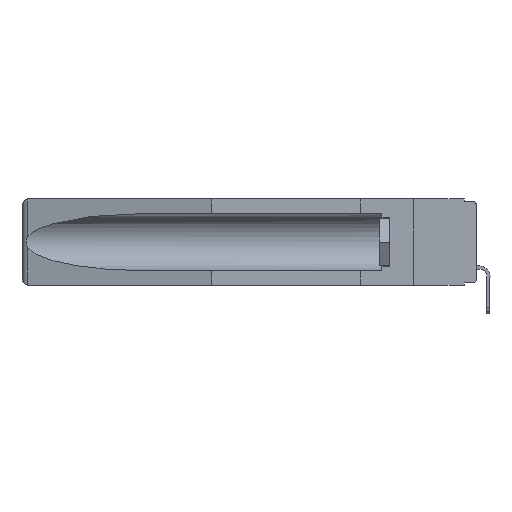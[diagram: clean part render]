
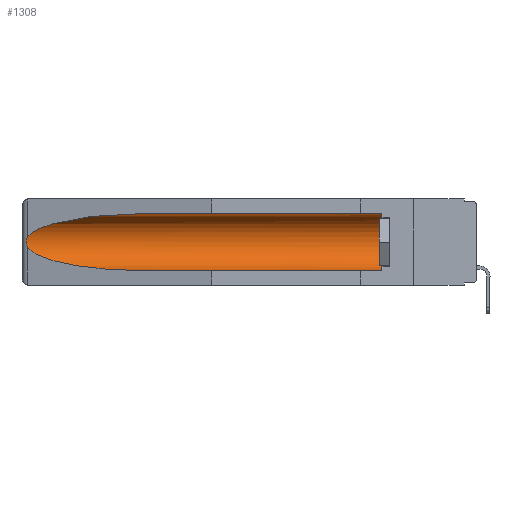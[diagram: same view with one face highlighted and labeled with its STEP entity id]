
A CAD part, left-side view. The second image highlights one B-rep face of the part: STEP entity #1308.
In plain terms, the highlighted cylindrical face has radius 2.857 mm (diameter 5.715 mm), a partial arc.
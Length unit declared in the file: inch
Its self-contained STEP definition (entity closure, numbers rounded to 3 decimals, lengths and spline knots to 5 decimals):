
#614 = ORIENTED_EDGE ( 'NONE', *, *, #19850, .T. ) ;
#837 = CARTESIAN_POINT ( 'NONE',  ( 0.26537, 1.52718, -0.19328 ) ) ;
#1308 = ADVANCED_FACE ( 'NONE', ( #6739 ), #22588, .F. ) ;
#1332 = EDGE_LOOP ( 'NONE', ( #6736, #7209, #614, #4670, #7236, #24581 ) ) ;
#2397 = VERTEX_POINT ( 'NONE', #21921 ) ;
#3023 = DIRECTION ( 'NONE',  ( 0., 0., 1. ) ) ;
#3344 = CARTESIAN_POINT ( 'NONE',  ( 0.155, 1.07973, -0.284 ) ) ;
#3628 = CARTESIAN_POINT ( 'NONE',  ( 0.21114, 1.30732, -0.284 ) ) ;
#4670 = ORIENTED_EDGE ( 'NONE', *, *, #9029, .F. ) ;
#4685 = AXIS2_PLACEMENT_3D ( 'NONE', #4795, #16959, #17043 ) ;
#4795 = CARTESIAN_POINT ( 'NONE',  ( 0.155, -0.30754, -0.1715 ) ) ;
#4807 = CARTESIAN_POINT ( 'NONE',  ( 0.26654, 1.53092, -0.15636 ) ) ;
#5540 = CARTESIAN_POINT ( 'NONE',  ( 0.155, 1.07973, -0.059 ) ) ;
#6115 = AXIS2_PLACEMENT_3D ( 'NONE', #7276, #15375, #3023 ) ;
#6623 = CARTESIAN_POINT ( 'NONE',  ( 0.26537, 1.52718, -0.14972 ) ) ;
#6736 = ORIENTED_EDGE ( 'NONE', *, *, #7638, .T. ) ;
#6739 = FACE_OUTER_BOUND ( 'NONE', #1332, .T. ) ;
#7209 = ORIENTED_EDGE ( 'NONE', *, *, #9747, .T. ) ;
#7236 = ORIENTED_EDGE ( 'NONE', *, *, #12128, .T. ) ;
#7238 = CARTESIAN_POINT ( 'NONE',  ( 0.155, 0.126, -0.059 ) ) ;
#7276 = CARTESIAN_POINT ( 'NONE',  ( 0.155, 0.126, -0.1715 ) ) ;
#7638 = EDGE_CURVE ( 'NONE', #10505, #26448, #10097, .T. ) ;
#7730 = VECTOR ( 'NONE', #8351, 39.37008 ) ;
#8350 = LINE ( 'NONE', #12063, #7730 ) ;
#8351 = DIRECTION ( 'NONE',  ( 0., 1., 0. ) ) ;
#8449 = CARTESIAN_POINT ( 'NONE',  ( 0.155, 1.07973, -0.284 ) ) ;
#9019 = VERTEX_POINT ( 'NONE', #7238 ) ;
#9029 = EDGE_CURVE ( 'NONE', #10270, #26548, #25011, .T. ) ;
#9129 = CARTESIAN_POINT ( 'NONE',  ( 0.26537, 1.52718, -0.14972 ) ) ;
#9357 = CARTESIAN_POINT ( 'NONE',  ( 0.21114, 1.30732, -0.059 ) ) ;
#9747 = EDGE_CURVE ( 'NONE', #26448, #2397, #12850, .T. ) ;
#9941 = CARTESIAN_POINT ( 'NONE',  ( 0.26537, 1.52718, -0.19328 ) ) ;
#10097 =( BOUNDED_CURVE ( )  B_SPLINE_CURVE ( 3, ( #17455, #9357, #14654, #6623 ),
 .UNSPECIFIED., .F., .T. ) 
 B_SPLINE_CURVE_WITH_KNOTS ( ( 4, 4 ),
 ( 4.71239, 6.08839 ),
 .UNSPECIFIED. ) 
 CURVE ( )  GEOMETRIC_REPRESENTATION_ITEM ( )  RATIONAL_B_SPLINE_CURVE ( ( 1., 0.848, 0.848, 1. ) ) 
 REPRESENTATION_ITEM ( '' )  );
#10270 = VERTEX_POINT ( 'NONE', #26228 ) ;
#10505 = VERTEX_POINT ( 'NONE', #5540 ) ;
#10785 = VECTOR ( 'NONE', #12995, 39.37008 ) ;
#10867 = CARTESIAN_POINT ( 'NONE',  ( 0.26655, 1.53094, -0.18657 ) ) ;
#12063 = CARTESIAN_POINT ( 'NONE',  ( 0.155, -0.30754, -0.059 ) ) ;
#12128 = EDGE_CURVE ( 'NONE', #10270, #9019, #15611, .T. ) ;
#12850 = B_SPLINE_CURVE_WITH_KNOTS ( 'NONE', 3,
 ( #9129, #23592, #4807, #25705, #13278, #13187, #21618, #10867, #25335, #837 ),
 .UNSPECIFIED., .F., .F.,
 ( 4, 2, 2, 2, 4 ),
 ( 0., 0.00029, 0.00058, 0.00087, 0.00117 ),
 .UNSPECIFIED. ) ;
#12995 = DIRECTION ( 'NONE',  ( 0., 1., 0. ) ) ;
#13187 = CARTESIAN_POINT ( 'NONE',  ( 0.2675, 1.53308, -0.17534 ) ) ;
#13278 = CARTESIAN_POINT ( 'NONE',  ( 0.2675, 1.53308, -0.16763 ) ) ;
#14654 = CARTESIAN_POINT ( 'NONE',  ( 0.25451, 1.48313, -0.09465 ) ) ;
#15375 = DIRECTION ( 'NONE',  ( 0., -1., 0. ) ) ;
#15611 = CIRCLE ( 'NONE', #6115, 0.1125 ) ;
#15881 = EDGE_CURVE ( 'NONE', #9019, #10505, #8350, .T. ) ;
#15953 = CARTESIAN_POINT ( 'NONE',  ( 0.25451, 1.48313, -0.24835 ) ) ;
#16959 = DIRECTION ( 'NONE',  ( 0., 1., 0. ) ) ;
#17043 = DIRECTION ( 'NONE',  ( 0., 0., 1. ) ) ;
#17455 = CARTESIAN_POINT ( 'NONE',  ( 0.155, 1.07973, -0.059 ) ) ;
#19850 = EDGE_CURVE ( 'NONE', #2397, #26548, #22654, .T. ) ;
#21618 = CARTESIAN_POINT ( 'NONE',  ( 0.2673, 1.53269, -0.17917 ) ) ;
#21921 = CARTESIAN_POINT ( 'NONE',  ( 0.26537, 1.52718, -0.19328 ) ) ;
#22588 = CYLINDRICAL_SURFACE ( 'NONE', #4685, 0.1125 ) ;
#22654 =( BOUNDED_CURVE ( )  B_SPLINE_CURVE ( 3, ( #9941, #15953, #3628, #3344 ),
 .UNSPECIFIED., .F., .F. ) 
 B_SPLINE_CURVE_WITH_KNOTS ( ( 4, 4 ),
 ( 0.1948, 1.5708 ),
 .UNSPECIFIED. ) 
 CURVE ( )  GEOMETRIC_REPRESENTATION_ITEM ( )  RATIONAL_B_SPLINE_CURVE ( ( 1., 0.848, 0.848, 1. ) ) 
 REPRESENTATION_ITEM ( '' )  );
#23047 = CARTESIAN_POINT ( 'NONE',  ( 0.155, -0.30754, -0.284 ) ) ;
#23592 = CARTESIAN_POINT ( 'NONE',  ( 0.26597, 1.52961, -0.15275 ) ) ;
#24581 = ORIENTED_EDGE ( 'NONE', *, *, #15881, .T. ) ;
#25011 = LINE ( 'NONE', #23047, #10785 ) ;
#25096 = CARTESIAN_POINT ( 'NONE',  ( 0.26537, 1.52718, -0.14972 ) ) ;
#25335 = CARTESIAN_POINT ( 'NONE',  ( 0.26597, 1.5296, -0.19026 ) ) ;
#25705 = CARTESIAN_POINT ( 'NONE',  ( 0.2673, 1.5327, -0.16383 ) ) ;
#26228 = CARTESIAN_POINT ( 'NONE',  ( 0.155, 0.126, -0.284 ) ) ;
#26448 = VERTEX_POINT ( 'NONE', #25096 ) ;
#26548 = VERTEX_POINT ( 'NONE', #8449 ) ;
